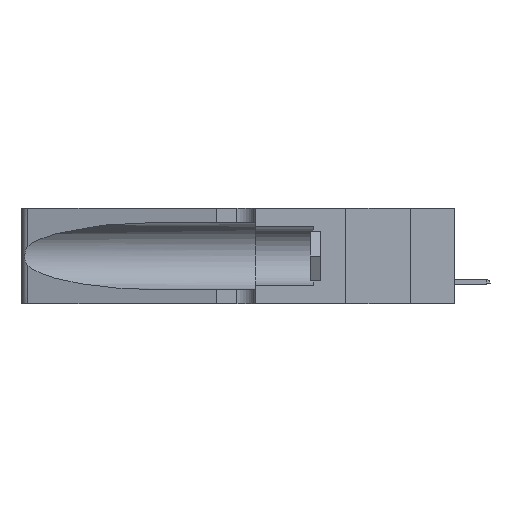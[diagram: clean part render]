
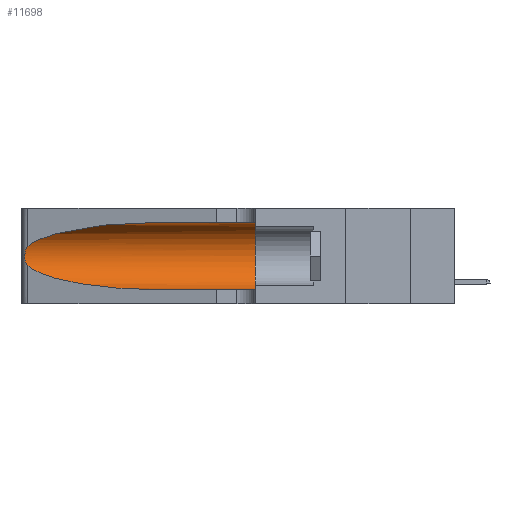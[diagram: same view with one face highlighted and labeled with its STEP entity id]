
A CAD part, left-side view. The second image highlights one B-rep face of the part: STEP entity #11698.
In plain terms, the highlighted cylindrical face has radius 3.308 mm (diameter 6.617 mm), a partial arc.
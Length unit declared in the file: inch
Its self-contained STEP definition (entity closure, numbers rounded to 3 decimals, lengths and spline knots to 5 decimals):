
#536 = DIRECTION ( 'NONE',  ( 0., -1., 0. ) ) ;
#678 = EDGE_CURVE ( 'NONE', #3457, #8367, #17188, .T. ) ;
#682 = CARTESIAN_POINT ( 'NONE',  ( 0.2373, 1.15595, 0.28018 ) ) ;
#1161 = CIRCLE ( 'NONE', #19361, 0.13025 ) ;
#2333 = EDGE_CURVE ( 'NONE', #24062, #8367, #1161, .T. ) ;
#2978 = CYLINDRICAL_SURFACE ( 'NONE', #23755, 0.13025 ) ;
#3457 = VERTEX_POINT ( 'NONE', #17695 ) ;
#3478 = CARTESIAN_POINT ( 'NONE',  ( 0.26017, 1.23833, 0.17102 ) ) ;
#4186 = CARTESIAN_POINT ( 'NONE',  ( 0.2373, 1.15595, 0.08982 ) ) ;
#4262 =( BOUNDED_CURVE ( )  B_SPLINE_CURVE ( 3, ( #8972, #4186, #13031, #17525 ),
 .UNSPECIFIED., .F., .F. ) 
 B_SPLINE_CURVE_WITH_KNOTS ( ( 4, 4 ),
 ( 3.44316, 4.71239 ),
 .UNSPECIFIED. ) 
 CURVE ( )  GEOMETRIC_REPRESENTATION_ITEM ( )  RATIONAL_B_SPLINE_CURVE ( ( 1., 0.87, 0.87, 1. ) ) 
 REPRESENTATION_ITEM ( '' )  );
#4460 = EDGE_LOOP ( 'NONE', ( #5784, #10320, #21020, #12971, #26747, #9906 ) ) ;
#5784 = ORIENTED_EDGE ( 'NONE', *, *, #19789, .T. ) ;
#6345 = VERTEX_POINT ( 'NONE', #20990 ) ;
#6370 = VERTEX_POINT ( 'NONE', #13797 ) ;
#7349 = FACE_OUTER_BOUND ( 'NONE', #4460, .T. ) ;
#7694 = CARTESIAN_POINT ( 'NONE',  ( 0.25555, 1.22994, 0.2215 ) ) ;
#8042 = CARTESIAN_POINT ( 'NONE',  ( 0.1305, 0.72297, 0.31525 ) ) ;
#8232 = DIRECTION ( 'NONE',  ( 0., 1., 0. ) ) ;
#8322 = VECTOR ( 'NONE', #536, 39.37008 ) ;
#8367 = VERTEX_POINT ( 'NONE', #26660 ) ;
#8972 = CARTESIAN_POINT ( 'NONE',  ( 0.25487, 1.22718, 0.14631 ) ) ;
#9091 = EDGE_CURVE ( 'NONE', #6345, #11131, #9922, .T. ) ;
#9906 = ORIENTED_EDGE ( 'NONE', *, *, #14661, .F. ) ;
#9922 = B_SPLINE_CURVE_WITH_KNOTS ( 'NONE', 3,
 ( #28252, #7694, #21497, #26288, #14567, #16826, #23887, #24026, #3478, #12624, #23727, #12335, #17274, #21791 ),
 .UNSPECIFIED., .F., .F.,
 ( 4, 2, 2, 2, 2, 2, 4 ),
 ( 0., 0.00027, 0.00053, 0.00107, 0.0016, 0.00187, 0.00214 ),
 .UNSPECIFIED. ) ;
#10320 = ORIENTED_EDGE ( 'NONE', *, *, #9091, .T. ) ;
#10877 = LINE ( 'NONE', #15224, #13566 ) ;
#11131 = VERTEX_POINT ( 'NONE', #24963 ) ;
#11698 = ADVANCED_FACE ( 'NONE', ( #7349 ), #2978, .F. ) ;
#12335 = CARTESIAN_POINT ( 'NONE',  ( 0.25639, 1.23186, 0.15144 ) ) ;
#12624 = CARTESIAN_POINT ( 'NONE',  ( 0.25856, 1.23593, 0.16098 ) ) ;
#12971 = ORIENTED_EDGE ( 'NONE', *, *, #678, .T. ) ;
#13031 = CARTESIAN_POINT ( 'NONE',  ( 0.18966, 0.96281, 0.05475 ) ) ;
#13181 = DIRECTION ( 'NONE',  ( 0., 0., 1. ) ) ;
#13566 = VECTOR ( 'NONE', #22136, 39.37008 ) ;
#13797 = CARTESIAN_POINT ( 'NONE',  ( 0.1305, 0.72297, 0.31525 ) ) ;
#14567 = CARTESIAN_POINT ( 'NONE',  ( 0.25854, 1.2359, 0.20912 ) ) ;
#14661 = EDGE_CURVE ( 'NONE', #6370, #24062, #10877, .T. ) ;
#15224 = CARTESIAN_POINT ( 'NONE',  ( 0.1305, 1.61858, 0.31525 ) ) ;
#16738 = CARTESIAN_POINT ( 'NONE',  ( 0.1305, 1.61858, 0.05475 ) ) ;
#16826 = CARTESIAN_POINT ( 'NONE',  ( 0.26018, 1.23835, 0.19895 ) ) ;
#17188 = LINE ( 'NONE', #16738, #8322 ) ;
#17274 = CARTESIAN_POINT ( 'NONE',  ( 0.25555, 1.22993, 0.14849 ) ) ;
#17525 = CARTESIAN_POINT ( 'NONE',  ( 0.1305, 0.72297, 0.05475 ) ) ;
#17695 = CARTESIAN_POINT ( 'NONE',  ( 0.1305, 0.72297, 0.05475 ) ) ;
#19215 =( BOUNDED_CURVE ( )  B_SPLINE_CURVE ( 3, ( #8042, #21236, #682, #21692 ),
 .UNSPECIFIED., .F., .T. ) 
 B_SPLINE_CURVE_WITH_KNOTS ( ( 4, 4 ),
 ( 1.5708, 2.84003 ),
 .UNSPECIFIED. ) 
 CURVE ( )  GEOMETRIC_REPRESENTATION_ITEM ( )  RATIONAL_B_SPLINE_CURVE ( ( 1., 0.87, 0.87, 1. ) ) 
 REPRESENTATION_ITEM ( '' )  );
#19323 = CARTESIAN_POINT ( 'NONE',  ( 0.1305, 1.61858, 0.185 ) ) ;
#19361 = AXIS2_PLACEMENT_3D ( 'NONE', #29377, #8232, #13181 ) ;
#19789 = EDGE_CURVE ( 'NONE', #6370, #6345, #19215, .T. ) ;
#20990 = CARTESIAN_POINT ( 'NONE',  ( 0.25487, 1.22718, 0.22369 ) ) ;
#21020 = ORIENTED_EDGE ( 'NONE', *, *, #22556, .T. ) ;
#21110 = CARTESIAN_POINT ( 'NONE',  ( 0.1305, 0.35, 0.31525 ) ) ;
#21236 = CARTESIAN_POINT ( 'NONE',  ( 0.18966, 0.96281, 0.31525 ) ) ;
#21497 = CARTESIAN_POINT ( 'NONE',  ( 0.25639, 1.23184, 0.21858 ) ) ;
#21692 = CARTESIAN_POINT ( 'NONE',  ( 0.25487, 1.22718, 0.22369 ) ) ;
#21791 = CARTESIAN_POINT ( 'NONE',  ( 0.25487, 1.22718, 0.14631 ) ) ;
#22136 = DIRECTION ( 'NONE',  ( 0., -1., 0. ) ) ;
#22556 = EDGE_CURVE ( 'NONE', #11131, #3457, #4262, .T. ) ;
#23677 = DIRECTION ( 'NONE',  ( 0., -1., 0. ) ) ;
#23727 = CARTESIAN_POINT ( 'NONE',  ( 0.25789, 1.23486, 0.15765 ) ) ;
#23755 = AXIS2_PLACEMENT_3D ( 'NONE', #19323, #23677, #26242 ) ;
#23887 = CARTESIAN_POINT ( 'NONE',  ( 0.26075, 1.23896, 0.19203 ) ) ;
#24026 = CARTESIAN_POINT ( 'NONE',  ( 0.26075, 1.23896, 0.178 ) ) ;
#24062 = VERTEX_POINT ( 'NONE', #21110 ) ;
#24963 = CARTESIAN_POINT ( 'NONE',  ( 0.25487, 1.22718, 0.14631 ) ) ;
#26242 = DIRECTION ( 'NONE',  ( 0., 0., -1. ) ) ;
#26288 = CARTESIAN_POINT ( 'NONE',  ( 0.25787, 1.23484, 0.2124 ) ) ;
#26660 = CARTESIAN_POINT ( 'NONE',  ( 0.1305, 0.35, 0.05475 ) ) ;
#26747 = ORIENTED_EDGE ( 'NONE', *, *, #2333, .F. ) ;
#28252 = CARTESIAN_POINT ( 'NONE',  ( 0.25487, 1.22718, 0.22369 ) ) ;
#29377 = CARTESIAN_POINT ( 'NONE',  ( 0.1305, 0.35, 0.185 ) ) ;
